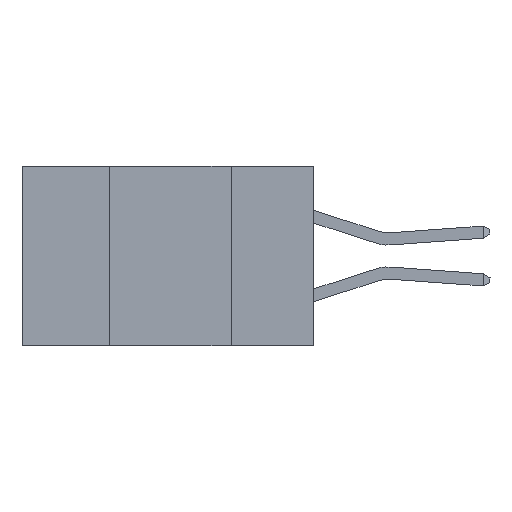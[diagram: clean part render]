
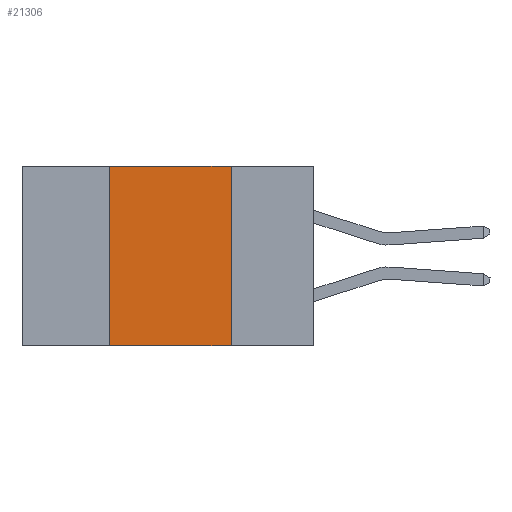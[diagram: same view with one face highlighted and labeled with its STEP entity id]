
A CAD part, left-side view. The second image highlights one B-rep face of the part: STEP entity #21306.
In plain terms, the highlighted planar face has unit normal (-1, 0, 0).
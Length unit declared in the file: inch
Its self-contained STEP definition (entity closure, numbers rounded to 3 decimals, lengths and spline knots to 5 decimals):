
#690 = VECTOR ( 'NONE', #6353, 39.37008 ) ;
#735 = CARTESIAN_POINT ( 'NONE',  ( 0., 0.42, 0. ) ) ;
#816 = EDGE_CURVE ( 'NONE', #6961, #12630, #17264, .T. ) ;
#1201 = CARTESIAN_POINT ( 'NONE',  ( 0., 0.6, 0. ) ) ;
#3038 = CARTESIAN_POINT ( 'NONE',  ( 0., 0.6, -0.37 ) ) ;
#3592 = CARTESIAN_POINT ( 'NONE',  ( 0., 0.17, 0. ) ) ;
#4131 = VERTEX_POINT ( 'NONE', #735 ) ;
#4935 = VECTOR ( 'NONE', #21450, 39.37008 ) ;
#5021 = CARTESIAN_POINT ( 'NONE',  ( 0., 0.17, -0.37 ) ) ;
#5732 = EDGE_CURVE ( 'NONE', #4131, #6961, #17438, .T. ) ;
#6353 = DIRECTION ( 'NONE',  ( 0., 0., -1. ) ) ;
#6961 = VERTEX_POINT ( 'NONE', #3592 ) ;
#7142 = DIRECTION ( 'NONE',  ( 0., 0., -1. ) ) ;
#7531 = EDGE_CURVE ( 'NONE', #9079, #12630, #23772, .T. ) ;
#8999 = EDGE_LOOP ( 'NONE', ( #12343, #15474, #15114, #12164 ) ) ;
#9079 = VERTEX_POINT ( 'NONE', #16305 ) ;
#10701 = PLANE ( 'NONE',  #17669 ) ;
#11295 = DIRECTION ( 'NONE',  ( 0., 0., 1. ) ) ;
#12032 = DIRECTION ( 'NONE',  ( 0., -1., 0. ) ) ;
#12164 = ORIENTED_EDGE ( 'NONE', *, *, #7531, .T. ) ;
#12343 = ORIENTED_EDGE ( 'NONE', *, *, #816, .F. ) ;
#12630 = VERTEX_POINT ( 'NONE', #5021 ) ;
#14005 = CARTESIAN_POINT ( 'NONE',  ( 0., 0.6, 0. ) ) ;
#15114 = ORIENTED_EDGE ( 'NONE', *, *, #17650, .F. ) ;
#15474 = ORIENTED_EDGE ( 'NONE', *, *, #5732, .F. ) ;
#15801 = FACE_OUTER_BOUND ( 'NONE', #8999, .T. ) ;
#16305 = CARTESIAN_POINT ( 'NONE',  ( 0., 0.42, -0.37 ) ) ;
#16375 = LINE ( 'NONE', #16698, #18100 ) ;
#16698 = CARTESIAN_POINT ( 'NONE',  ( 0., 0.42, 0. ) ) ;
#16758 = VECTOR ( 'NONE', #12032, 39.37008 ) ;
#17264 = LINE ( 'NONE', #17393, #690 ) ;
#17393 = CARTESIAN_POINT ( 'NONE',  ( 0., 0.17, 0. ) ) ;
#17438 = LINE ( 'NONE', #14005, #4935 ) ;
#17650 = EDGE_CURVE ( 'NONE', #9079, #4131, #16375, .T. ) ;
#17669 = AXIS2_PLACEMENT_3D ( 'NONE', #1201, #21691, #7142 ) ;
#18100 = VECTOR ( 'NONE', #11295, 39.37008 ) ;
#21306 = ADVANCED_FACE ( 'NONE', ( #15801 ), #10701, .F. ) ;
#21450 = DIRECTION ( 'NONE',  ( 0., -1., 0. ) ) ;
#21691 = DIRECTION ( 'NONE',  ( 1., 0., 0. ) ) ;
#23772 = LINE ( 'NONE', #3038, #16758 ) ;
